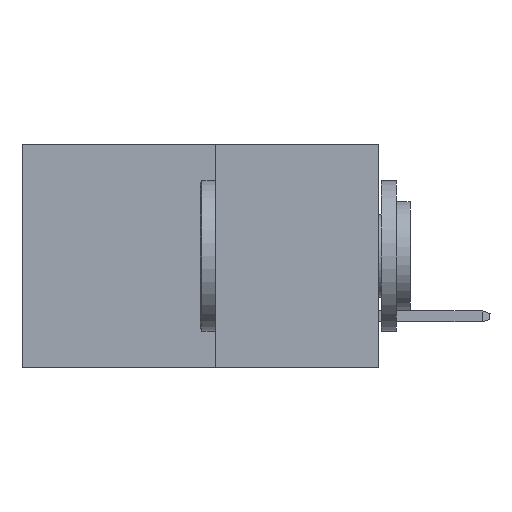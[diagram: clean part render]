
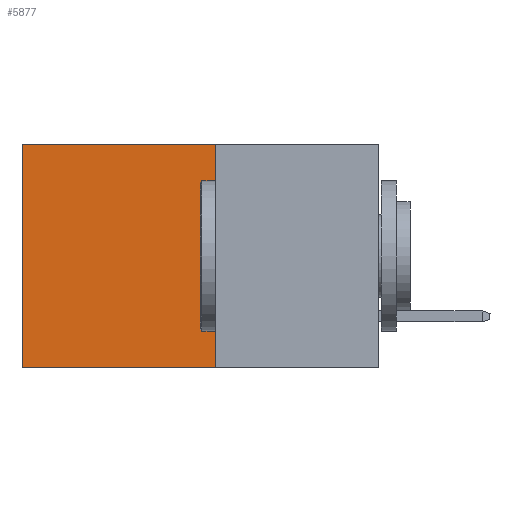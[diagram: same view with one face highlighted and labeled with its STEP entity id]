
A CAD part, left-side view. The second image highlights one B-rep face of the part: STEP entity #5877.
In plain terms, the highlighted planar face has unit normal (-1, 0, 0).
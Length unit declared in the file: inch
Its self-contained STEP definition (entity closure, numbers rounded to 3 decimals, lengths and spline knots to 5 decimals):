
#337 = CARTESIAN_POINT ( 'NONE',  ( 0.277, 0.27, 0. ) ) ;
#377 = DIRECTION ( 'NONE',  ( 0., 0., -1. ) ) ;
#378 = DIRECTION ( 'NONE',  ( 1., 0., 0. ) ) ;
#541 = CARTESIAN_POINT ( 'NONE',  ( 0.277, 0.27, -0.37 ) ) ;
#690 = PLANE ( 'NONE',  #11111 ) ;
#832 = ORIENTED_EDGE ( 'NONE', *, *, #1901, .F. ) ;
#962 = DIRECTION ( 'NONE',  ( 0., 0., -1. ) ) ;
#1282 = LINE ( 'NONE', #10222, #10333 ) ;
#1556 = CARTESIAN_POINT ( 'NONE',  ( 0.277, 0.27, -0.37 ) ) ;
#1582 = VECTOR ( 'NONE', #3238, 39.37008 ) ;
#1901 = EDGE_CURVE ( 'NONE', #2412, #5651, #7773, .T. ) ;
#2246 = CARTESIAN_POINT ( 'NONE',  ( 0.277, 0.27, -0.37 ) ) ;
#2412 = VERTEX_POINT ( 'NONE', #10806 ) ;
#2444 = DIRECTION ( 'NONE',  ( 0., 1., 0. ) ) ;
#3238 = DIRECTION ( 'NONE',  ( 0., 0., -1. ) ) ;
#3251 = CARTESIAN_POINT ( 'NONE',  ( 0.277, 0.59, -0.37 ) ) ;
#3562 = ORIENTED_EDGE ( 'NONE', *, *, #8017, .T. ) ;
#3883 = CARTESIAN_POINT ( 'NONE',  ( 0.277, 0.59, -0.37 ) ) ;
#4149 = EDGE_LOOP ( 'NONE', ( #7876, #10241, #832, #3562 ) ) ;
#4822 = EDGE_CURVE ( 'NONE', #5651, #7108, #1282, .T. ) ;
#5458 = EDGE_CURVE ( 'NONE', #8888, #7108, #8981, .T. ) ;
#5651 = VERTEX_POINT ( 'NONE', #2246 ) ;
#5877 = ADVANCED_FACE ( 'NONE', ( #8606 ), #690, .F. ) ;
#7108 = VERTEX_POINT ( 'NONE', #3883 ) ;
#7199 = CARTESIAN_POINT ( 'NONE',  ( 0.277, 0.59, 0. ) ) ;
#7484 = VECTOR ( 'NONE', #962, 39.37008 ) ;
#7773 = LINE ( 'NONE', #1556, #7484 ) ;
#7876 = ORIENTED_EDGE ( 'NONE', *, *, #5458, .T. ) ;
#8017 = EDGE_CURVE ( 'NONE', #2412, #8888, #11363, .T. ) ;
#8606 = FACE_OUTER_BOUND ( 'NONE', #4149, .T. ) ;
#8888 = VERTEX_POINT ( 'NONE', #7199 ) ;
#8981 = LINE ( 'NONE', #3251, #1582 ) ;
#9321 = VECTOR ( 'NONE', #2444, 39.37008 ) ;
#10066 = DIRECTION ( 'NONE',  ( 0., 1., 0. ) ) ;
#10222 = CARTESIAN_POINT ( 'NONE',  ( 0.277, 0.27, -0.37 ) ) ;
#10241 = ORIENTED_EDGE ( 'NONE', *, *, #4822, .F. ) ;
#10333 = VECTOR ( 'NONE', #10066, 39.37008 ) ;
#10806 = CARTESIAN_POINT ( 'NONE',  ( 0.277, 0.27, 0. ) ) ;
#11111 = AXIS2_PLACEMENT_3D ( 'NONE', #541, #378, #377 ) ;
#11363 = LINE ( 'NONE', #337, #9321 ) ;
